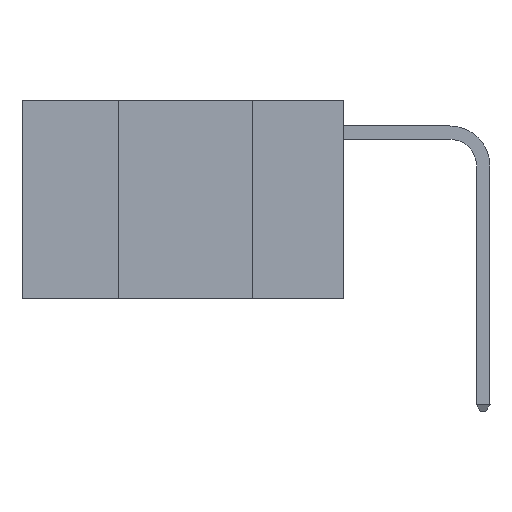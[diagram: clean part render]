
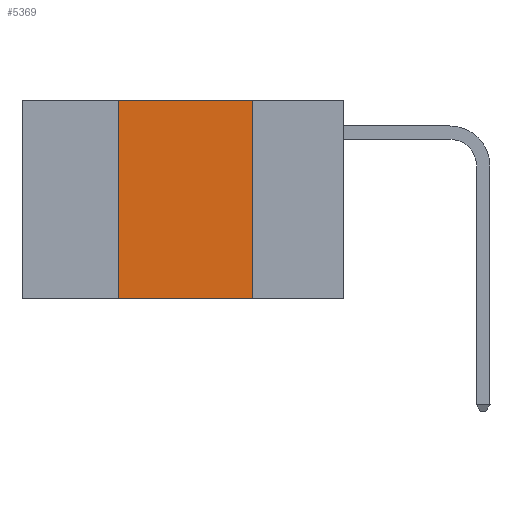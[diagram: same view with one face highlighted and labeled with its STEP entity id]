
A CAD part, left-side view. The second image highlights one B-rep face of the part: STEP entity #5369.
In plain terms, the highlighted planar face has unit normal (-1, 0, 0).
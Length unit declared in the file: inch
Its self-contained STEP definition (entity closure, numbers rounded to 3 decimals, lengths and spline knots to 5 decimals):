
#90 = EDGE_CURVE ( 'NONE', #4940, #4841, #7062, .T. ) ;
#220 = CARTESIAN_POINT ( 'NONE',  ( 0., 0.6, -0.37 ) ) ;
#226 = EDGE_CURVE ( 'NONE', #4368, #4841, #2849, .T. ) ;
#728 = VECTOR ( 'NONE', #1025, 39.37008 ) ;
#951 = LINE ( 'NONE', #3057, #995 ) ;
#995 = VECTOR ( 'NONE', #2869, 39.37008 ) ;
#1025 = DIRECTION ( 'NONE',  ( 0., -1., 0. ) ) ;
#1219 = CARTESIAN_POINT ( 'NONE',  ( 0., 0.6, 0. ) ) ;
#1290 = DIRECTION ( 'NONE',  ( 0., 0., -1. ) ) ;
#1392 = PLANE ( 'NONE',  #6297 ) ;
#1505 = CARTESIAN_POINT ( 'NONE',  ( 0., 0.6, 0. ) ) ;
#1531 = ORIENTED_EDGE ( 'NONE', *, *, #226, .F. ) ;
#1552 = DIRECTION ( 'NONE',  ( 1., 0., 0. ) ) ;
#1882 = EDGE_LOOP ( 'NONE', ( #1531, #4427, #6765, #7801 ) ) ;
#2300 = LINE ( 'NONE', #1219, #728 ) ;
#2681 = VECTOR ( 'NONE', #8165, 39.37008 ) ;
#2849 = LINE ( 'NONE', #7442, #2681 ) ;
#2869 = DIRECTION ( 'NONE',  ( 0., 0., 1. ) ) ;
#3057 = CARTESIAN_POINT ( 'NONE',  ( 0., 0.42, 0. ) ) ;
#4012 = DIRECTION ( 'NONE',  ( 0., -1., 0. ) ) ;
#4368 = VERTEX_POINT ( 'NONE', #5481 ) ;
#4427 = ORIENTED_EDGE ( 'NONE', *, *, #7089, .F. ) ;
#4841 = VERTEX_POINT ( 'NONE', #5793 ) ;
#4940 = VERTEX_POINT ( 'NONE', #5094 ) ;
#5094 = CARTESIAN_POINT ( 'NONE',  ( 0., 0.42, -0.37 ) ) ;
#5369 = ADVANCED_FACE ( 'NONE', ( #8434 ), #1392, .F. ) ;
#5481 = CARTESIAN_POINT ( 'NONE',  ( 0., 0.17, 0. ) ) ;
#5793 = CARTESIAN_POINT ( 'NONE',  ( 0., 0.17, -0.37 ) ) ;
#6297 = AXIS2_PLACEMENT_3D ( 'NONE', #1505, #1552, #1290 ) ;
#6343 = CARTESIAN_POINT ( 'NONE',  ( 0., 0.42, 0. ) ) ;
#6765 = ORIENTED_EDGE ( 'NONE', *, *, #6855, .F. ) ;
#6855 = EDGE_CURVE ( 'NONE', #4940, #8387, #951, .T. ) ;
#7062 = LINE ( 'NONE', #220, #7162 ) ;
#7089 = EDGE_CURVE ( 'NONE', #8387, #4368, #2300, .T. ) ;
#7162 = VECTOR ( 'NONE', #4012, 39.37008 ) ;
#7442 = CARTESIAN_POINT ( 'NONE',  ( 0., 0.17, 0. ) ) ;
#7801 = ORIENTED_EDGE ( 'NONE', *, *, #90, .T. ) ;
#8165 = DIRECTION ( 'NONE',  ( 0., 0., -1. ) ) ;
#8387 = VERTEX_POINT ( 'NONE', #6343 ) ;
#8434 = FACE_OUTER_BOUND ( 'NONE', #1882, .T. ) ;
